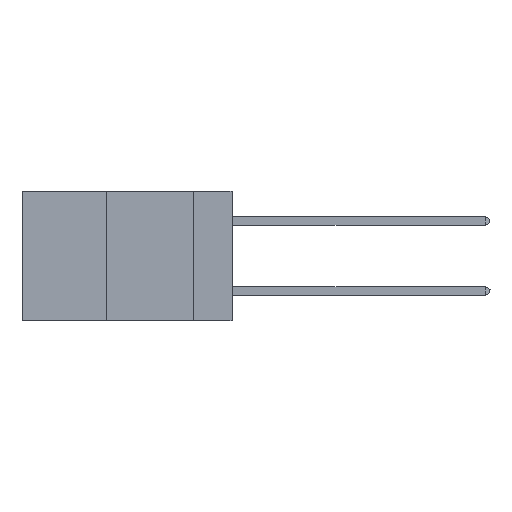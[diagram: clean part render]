
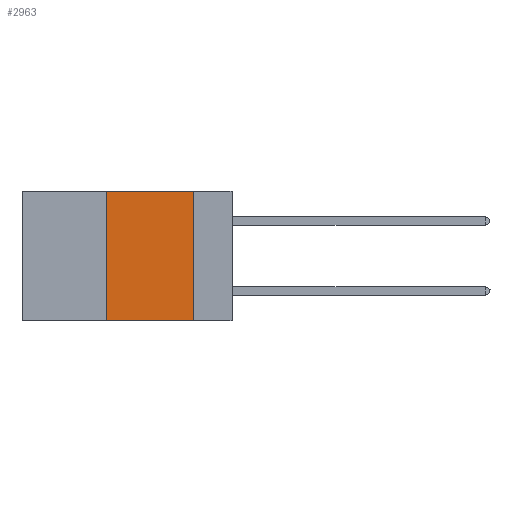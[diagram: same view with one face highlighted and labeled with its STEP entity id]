
A CAD part, left-side view. The second image highlights one B-rep face of the part: STEP entity #2963.
In plain terms, the highlighted planar face has unit normal (-1, 0, 0).
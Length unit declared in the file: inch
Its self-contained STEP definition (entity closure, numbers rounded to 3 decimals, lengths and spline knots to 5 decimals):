
#892 = CARTESIAN_POINT ( 'NONE',  ( 0., 0.36, 0. ) ) ;
#1435 = EDGE_CURVE ( 'NONE', #7054, #6050, #25005, .T. ) ;
#2963 = ADVANCED_FACE ( 'NONE', ( #3971 ), #4613, .F. ) ;
#3971 = FACE_OUTER_BOUND ( 'NONE', #15329, .T. ) ;
#4080 = CARTESIAN_POINT ( 'NONE',  ( 0., 0.6, 0. ) ) ;
#4202 = CARTESIAN_POINT ( 'NONE',  ( 0., 0.6, -0.37 ) ) ;
#4613 = PLANE ( 'NONE',  #20264 ) ;
#4750 = DIRECTION ( 'NONE',  ( 0., 0., 1. ) ) ;
#5268 = CARTESIAN_POINT ( 'NONE',  ( 0., 0.11, -0.37 ) ) ;
#5684 = ORIENTED_EDGE ( 'NONE', *, *, #11448, .F. ) ;
#6050 = VERTEX_POINT ( 'NONE', #26345 ) ;
#6136 = ORIENTED_EDGE ( 'NONE', *, *, #1435, .F. ) ;
#6688 = DIRECTION ( 'NONE',  ( 0., 0., -1. ) ) ;
#7054 = VERTEX_POINT ( 'NONE', #19431 ) ;
#7237 = VECTOR ( 'NONE', #4750, 39.37008 ) ;
#8973 = ORIENTED_EDGE ( 'NONE', *, *, #26501, .T. ) ;
#10379 = CARTESIAN_POINT ( 'NONE',  ( 0., 0.11, 0. ) ) ;
#10863 = LINE ( 'NONE', #4202, #26993 ) ;
#10915 = CARTESIAN_POINT ( 'NONE',  ( 0., 0.6, 0. ) ) ;
#11448 = EDGE_CURVE ( 'NONE', #6050, #21379, #13319, .T. ) ;
#13319 = LINE ( 'NONE', #4080, #22578 ) ;
#13548 = CARTESIAN_POINT ( 'NONE',  ( 0., 0.11, 0. ) ) ;
#14396 = DIRECTION ( 'NONE',  ( 0., -1., 0. ) ) ;
#15329 = EDGE_LOOP ( 'NONE', ( #17632, #5684, #6136, #8973 ) ) ;
#15534 = VERTEX_POINT ( 'NONE', #5268 ) ;
#16661 = DIRECTION ( 'NONE',  ( 0., -1., 0. ) ) ;
#17632 = ORIENTED_EDGE ( 'NONE', *, *, #18853, .F. ) ;
#18853 = EDGE_CURVE ( 'NONE', #21379, #15534, #25544, .T. ) ;
#19431 = CARTESIAN_POINT ( 'NONE',  ( 0., 0.36, -0.37 ) ) ;
#20032 = VECTOR ( 'NONE', #23276, 39.37008 ) ;
#20264 = AXIS2_PLACEMENT_3D ( 'NONE', #10915, #25634, #6688 ) ;
#21379 = VERTEX_POINT ( 'NONE', #13548 ) ;
#22578 = VECTOR ( 'NONE', #14396, 39.37008 ) ;
#23276 = DIRECTION ( 'NONE',  ( 0., 0., -1. ) ) ;
#25005 = LINE ( 'NONE', #892, #7237 ) ;
#25544 = LINE ( 'NONE', #10379, #20032 ) ;
#25634 = DIRECTION ( 'NONE',  ( 1., 0., 0. ) ) ;
#26345 = CARTESIAN_POINT ( 'NONE',  ( 0., 0.36, 0. ) ) ;
#26501 = EDGE_CURVE ( 'NONE', #7054, #15534, #10863, .T. ) ;
#26993 = VECTOR ( 'NONE', #16661, 39.37008 ) ;
